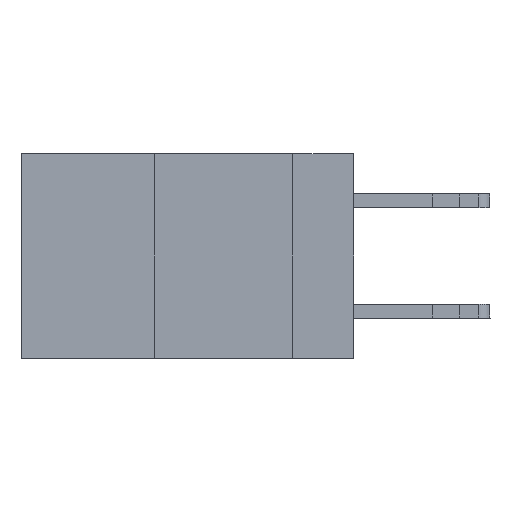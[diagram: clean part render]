
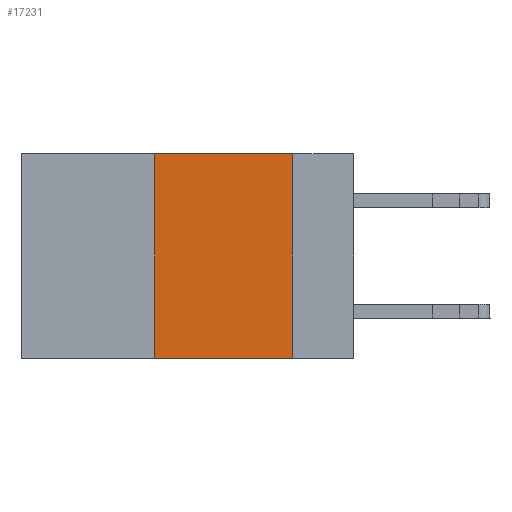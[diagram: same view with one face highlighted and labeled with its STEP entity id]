
A CAD part, left-side view. The second image highlights one B-rep face of the part: STEP entity #17231.
In plain terms, the highlighted planar face has unit normal (-1, 0, 0).
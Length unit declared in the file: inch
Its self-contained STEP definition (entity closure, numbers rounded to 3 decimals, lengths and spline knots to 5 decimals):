
#1529 = AXIS2_PLACEMENT_3D ( 'NONE', #3317, #13380, #4784 ) ;
#2214 = VECTOR ( 'NONE', #7959, 39.37008 ) ;
#2984 = FACE_OUTER_BOUND ( 'NONE', #6283, .T. ) ;
#3317 = CARTESIAN_POINT ( 'NONE',  ( 0., 0.6, 0. ) ) ;
#3418 = VERTEX_POINT ( 'NONE', #8259 ) ;
#4104 = EDGE_CURVE ( 'NONE', #6138, #4930, #10342, .T. ) ;
#4784 = DIRECTION ( 'NONE',  ( 0., 0., -1. ) ) ;
#4789 = VECTOR ( 'NONE', #9441, 39.37008 ) ;
#4864 = VECTOR ( 'NONE', #15462, 39.37008 ) ;
#4930 = VERTEX_POINT ( 'NONE', #13020 ) ;
#5439 = CARTESIAN_POINT ( 'NONE',  ( 0., 0.6, -0.37 ) ) ;
#6138 = VERTEX_POINT ( 'NONE', #8410 ) ;
#6283 = EDGE_LOOP ( 'NONE', ( #7357, #7652, #8026, #8763 ) ) ;
#7357 = ORIENTED_EDGE ( 'NONE', *, *, #4104, .F. ) ;
#7652 = ORIENTED_EDGE ( 'NONE', *, *, #10333, .F. ) ;
#7959 = DIRECTION ( 'NONE',  ( 0., 0., -1. ) ) ;
#8026 = ORIENTED_EDGE ( 'NONE', *, *, #16296, .F. ) ;
#8259 = CARTESIAN_POINT ( 'NONE',  ( 0., 0.36, 0. ) ) ;
#8410 = CARTESIAN_POINT ( 'NONE',  ( 0., 0.11, 0. ) ) ;
#8552 = LINE ( 'NONE', #13731, #4789 ) ;
#8591 = DIRECTION ( 'NONE',  ( 0., 0., 1. ) ) ;
#8763 = ORIENTED_EDGE ( 'NONE', *, *, #14757, .T. ) ;
#9441 = DIRECTION ( 'NONE',  ( 0., -1., 0. ) ) ;
#9986 = LINE ( 'NONE', #12894, #16761 ) ;
#10333 = EDGE_CURVE ( 'NONE', #3418, #6138, #8552, .T. ) ;
#10342 = LINE ( 'NONE', #16713, #2214 ) ;
#12894 = CARTESIAN_POINT ( 'NONE',  ( 0., 0.36, 0. ) ) ;
#13020 = CARTESIAN_POINT ( 'NONE',  ( 0., 0.11, -0.37 ) ) ;
#13380 = DIRECTION ( 'NONE',  ( 1., 0., 0. ) ) ;
#13395 = LINE ( 'NONE', #5439, #4864 ) ;
#13731 = CARTESIAN_POINT ( 'NONE',  ( 0., 0.6, 0. ) ) ;
#14757 = EDGE_CURVE ( 'NONE', #16331, #4930, #13395, .T. ) ;
#14802 = PLANE ( 'NONE',  #1529 ) ;
#15462 = DIRECTION ( 'NONE',  ( 0., -1., 0. ) ) ;
#15891 = CARTESIAN_POINT ( 'NONE',  ( 0., 0.36, -0.37 ) ) ;
#16296 = EDGE_CURVE ( 'NONE', #16331, #3418, #9986, .T. ) ;
#16331 = VERTEX_POINT ( 'NONE', #15891 ) ;
#16713 = CARTESIAN_POINT ( 'NONE',  ( 0., 0.11, 0. ) ) ;
#16761 = VECTOR ( 'NONE', #8591, 39.37008 ) ;
#17231 = ADVANCED_FACE ( 'NONE', ( #2984 ), #14802, .F. ) ;
